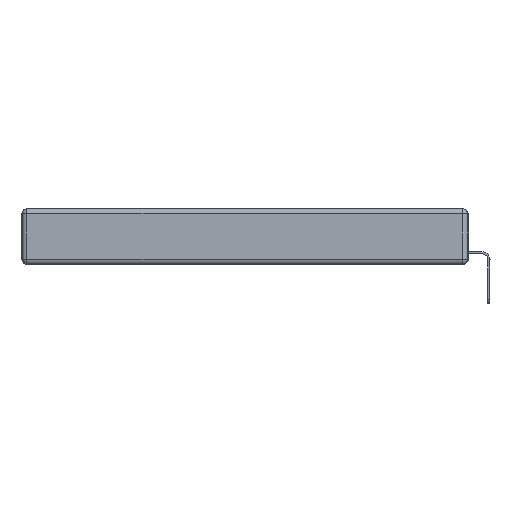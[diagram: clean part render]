
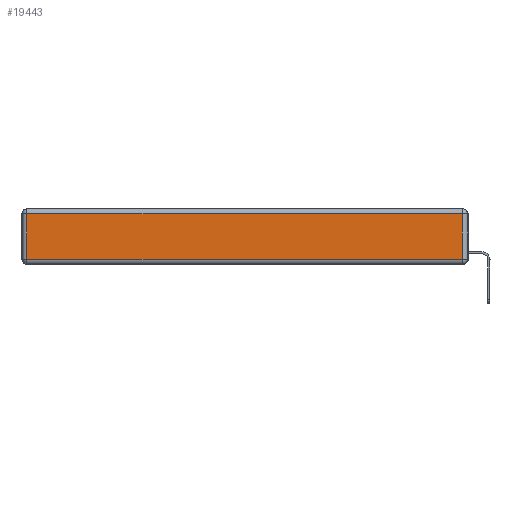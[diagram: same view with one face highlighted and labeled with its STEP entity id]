
A CAD part, left-side view. The second image highlights one B-rep face of the part: STEP entity #19443.
In plain terms, the highlighted planar face has unit normal (-1, 0, 0).
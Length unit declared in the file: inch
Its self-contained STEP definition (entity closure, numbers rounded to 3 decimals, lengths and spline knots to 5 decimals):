
#1378 = DIRECTION ( 'NONE',  ( 0., 0., 1. ) ) ;
#1631 = VERTEX_POINT ( 'NONE', #4118 ) ;
#2746 = LINE ( 'NONE', #5436, #19713 ) ;
#3936 = LINE ( 'NONE', #15277, #20885 ) ;
#4118 = CARTESIAN_POINT ( 'NONE',  ( 0., 0.03, -0.313 ) ) ;
#4125 = FACE_OUTER_BOUND ( 'NONE', #17226, .T. ) ;
#5204 = CARTESIAN_POINT ( 'NONE',  ( 0., 2.72, -0.313 ) ) ;
#5436 = CARTESIAN_POINT ( 'NONE',  ( 0., 2.72, -0.343 ) ) ;
#5556 = DIRECTION ( 'NONE',  ( 0., 1., 0. ) ) ;
#5829 = EDGE_CURVE ( 'NONE', #17168, #10924, #2746, .T. ) ;
#5981 = ORIENTED_EDGE ( 'NONE', *, *, #9977, .T. ) ;
#6248 = PLANE ( 'NONE',  #10127 ) ;
#6637 = LINE ( 'NONE', #12084, #9510 ) ;
#6864 = LINE ( 'NONE', #19565, #9222 ) ;
#7028 = CARTESIAN_POINT ( 'NONE',  ( 0., 2.72, -0.03 ) ) ;
#7768 = CARTESIAN_POINT ( 'NONE',  ( 0., 0., -0.343 ) ) ;
#9222 = VECTOR ( 'NONE', #9839, 39.37008 ) ;
#9510 = VECTOR ( 'NONE', #20753, 39.37008 ) ;
#9839 = DIRECTION ( 'NONE',  ( 0., 0., 1. ) ) ;
#9977 = EDGE_CURVE ( 'NONE', #10924, #1631, #6637, .T. ) ;
#10127 = AXIS2_PLACEMENT_3D ( 'NONE', #7768, #14551, #1378 ) ;
#10924 = VERTEX_POINT ( 'NONE', #5204 ) ;
#11909 = EDGE_CURVE ( 'NONE', #1631, #21037, #6864, .T. ) ;
#12084 = CARTESIAN_POINT ( 'NONE',  ( 0., 0., -0.313 ) ) ;
#14493 = EDGE_CURVE ( 'NONE', #21037, #17168, #3936, .T. ) ;
#14551 = DIRECTION ( 'NONE',  ( -1., 0., 0. ) ) ;
#14833 = CARTESIAN_POINT ( 'NONE',  ( 0., 0.03, -0.03 ) ) ;
#15025 = DIRECTION ( 'NONE',  ( 0., 0., -1. ) ) ;
#15277 = CARTESIAN_POINT ( 'NONE',  ( 0., 2.75, -0.03 ) ) ;
#17168 = VERTEX_POINT ( 'NONE', #7028 ) ;
#17226 = EDGE_LOOP ( 'NONE', ( #5981, #19576, #20828, #19983 ) ) ;
#19443 = ADVANCED_FACE ( 'NONE', ( #4125 ), #6248, .T. ) ;
#19565 = CARTESIAN_POINT ( 'NONE',  ( 0., 0.03, -0.343 ) ) ;
#19576 = ORIENTED_EDGE ( 'NONE', *, *, #11909, .T. ) ;
#19713 = VECTOR ( 'NONE', #15025, 39.37008 ) ;
#19983 = ORIENTED_EDGE ( 'NONE', *, *, #5829, .T. ) ;
#20753 = DIRECTION ( 'NONE',  ( 0., -1., 0. ) ) ;
#20828 = ORIENTED_EDGE ( 'NONE', *, *, #14493, .T. ) ;
#20885 = VECTOR ( 'NONE', #5556, 39.37008 ) ;
#21037 = VERTEX_POINT ( 'NONE', #14833 ) ;
